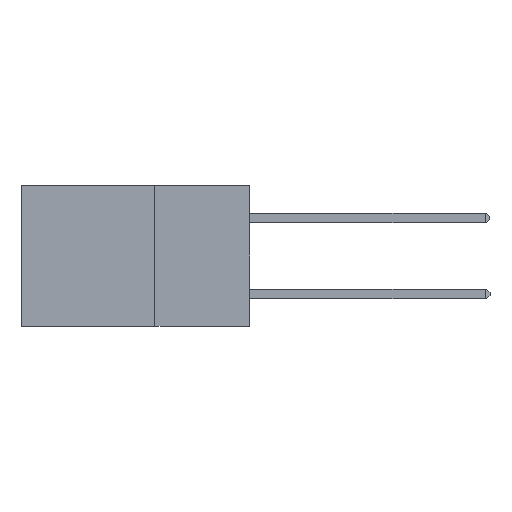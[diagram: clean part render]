
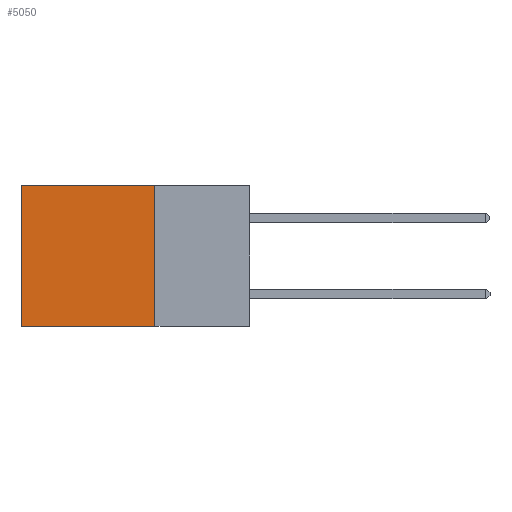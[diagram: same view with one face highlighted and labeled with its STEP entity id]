
A CAD part, left-side view. The second image highlights one B-rep face of the part: STEP entity #5050.
In plain terms, the highlighted planar face has unit normal (-1, 0, 0).
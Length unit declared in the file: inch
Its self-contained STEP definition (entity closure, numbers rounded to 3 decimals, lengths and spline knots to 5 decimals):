
#1667 = ORIENTED_EDGE ( 'NONE', *, *, #9501, .T. ) ;
#1836 = VERTEX_POINT ( 'NONE', #4321 ) ;
#3196 = EDGE_CURVE ( 'NONE', #7154, #4796, #10348, .T. ) ;
#3923 = DIRECTION ( 'NONE',  ( 0., 1., 0. ) ) ;
#4321 = CARTESIAN_POINT ( 'NONE',  ( 0.2875, 0.6, 0. ) ) ;
#4386 = PLANE ( 'NONE',  #13013 ) ;
#4595 = CARTESIAN_POINT ( 'NONE',  ( 0.2875, 0.25, 0. ) ) ;
#4796 = VERTEX_POINT ( 'NONE', #16290 ) ;
#4995 = EDGE_LOOP ( 'NONE', ( #1667, #20227, #13699, #6057 ) ) ;
#5050 = ADVANCED_FACE ( 'NONE', ( #13354 ), #4386, .F. ) ;
#5411 = DIRECTION ( 'NONE',  ( 0., 1., 0. ) ) ;
#5473 = CARTESIAN_POINT ( 'NONE',  ( 0.2875, 0.25, 0. ) ) ;
#5961 = DIRECTION ( 'NONE',  ( 1., 0., 0. ) ) ;
#6057 = ORIENTED_EDGE ( 'NONE', *, *, #18533, .T. ) ;
#7154 = VERTEX_POINT ( 'NONE', #14144 ) ;
#7297 = LINE ( 'NONE', #14920, #15641 ) ;
#8713 = CARTESIAN_POINT ( 'NONE',  ( 0.2875, 0.6, 0. ) ) ;
#8739 = VERTEX_POINT ( 'NONE', #19223 ) ;
#8928 = LINE ( 'NONE', #5473, #20523 ) ;
#9501 = EDGE_CURVE ( 'NONE', #1836, #8739, #18666, .T. ) ;
#10154 = EDGE_CURVE ( 'NONE', #4796, #8739, #7297, .T. ) ;
#10348 = LINE ( 'NONE', #4595, #13551 ) ;
#11859 = DIRECTION ( 'NONE',  ( 0., 0., -1. ) ) ;
#13013 = AXIS2_PLACEMENT_3D ( 'NONE', #13778, #5961, #16994 ) ;
#13354 = FACE_OUTER_BOUND ( 'NONE', #4995, .T. ) ;
#13551 = VECTOR ( 'NONE', #17194, 39.37008 ) ;
#13699 = ORIENTED_EDGE ( 'NONE', *, *, #3196, .F. ) ;
#13778 = CARTESIAN_POINT ( 'NONE',  ( 0.2875, 0.25, 0. ) ) ;
#14144 = CARTESIAN_POINT ( 'NONE',  ( 0.2875, 0.25, 0. ) ) ;
#14433 = VECTOR ( 'NONE', #11859, 39.37008 ) ;
#14920 = CARTESIAN_POINT ( 'NONE',  ( 0.2875, 0.25, -0.37 ) ) ;
#15641 = VECTOR ( 'NONE', #3923, 39.37008 ) ;
#16290 = CARTESIAN_POINT ( 'NONE',  ( 0.2875, 0.25, -0.37 ) ) ;
#16994 = DIRECTION ( 'NONE',  ( 0., 0., -1. ) ) ;
#17194 = DIRECTION ( 'NONE',  ( 0., 0., -1. ) ) ;
#18533 = EDGE_CURVE ( 'NONE', #7154, #1836, #8928, .T. ) ;
#18666 = LINE ( 'NONE', #8713, #14433 ) ;
#19223 = CARTESIAN_POINT ( 'NONE',  ( 0.2875, 0.6, -0.37 ) ) ;
#20227 = ORIENTED_EDGE ( 'NONE', *, *, #10154, .F. ) ;
#20523 = VECTOR ( 'NONE', #5411, 39.37008 ) ;
